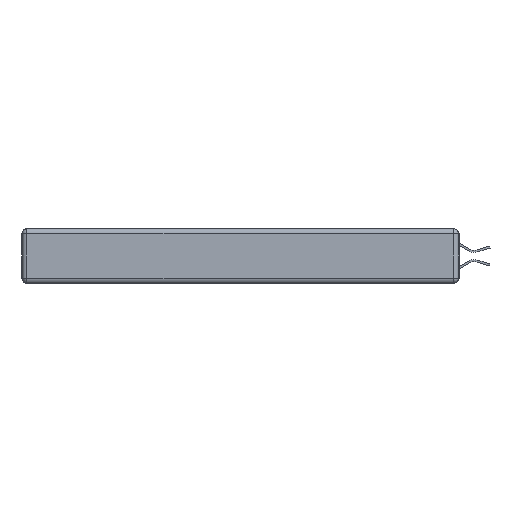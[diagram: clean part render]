
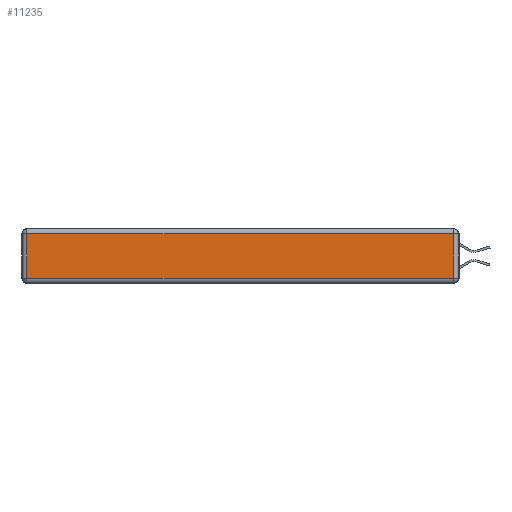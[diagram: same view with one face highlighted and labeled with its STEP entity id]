
A CAD part, left-side view. The second image highlights one B-rep face of the part: STEP entity #11235.
In plain terms, the highlighted planar face has unit normal (-1, 0, 0).
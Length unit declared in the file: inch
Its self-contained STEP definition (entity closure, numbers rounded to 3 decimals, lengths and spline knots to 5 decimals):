
#348 = VERTEX_POINT ( 'NONE', #9298 ) ;
#1305 = LINE ( 'NONE', #13973, #2367 ) ;
#1546 = ORIENTED_EDGE ( 'NONE', *, *, #17065, .T. ) ;
#2367 = VECTOR ( 'NONE', #12504, 39.37008 ) ;
#2488 = PLANE ( 'NONE',  #15989 ) ;
#2818 = VERTEX_POINT ( 'NONE', #19683 ) ;
#3318 = LINE ( 'NONE', #5672, #21257 ) ;
#3895 = FACE_OUTER_BOUND ( 'NONE', #20191, .T. ) ;
#5672 = CARTESIAN_POINT ( 'NONE',  ( 0., 2.75, -0.03 ) ) ;
#5924 = ORIENTED_EDGE ( 'NONE', *, *, #8957, .T. ) ;
#7052 = CARTESIAN_POINT ( 'NONE',  ( 0., 0., -0.313 ) ) ;
#7129 = DIRECTION ( 'NONE',  ( 0., -1., 0. ) ) ;
#7643 = ORIENTED_EDGE ( 'NONE', *, *, #12634, .T. ) ;
#8957 = EDGE_CURVE ( 'NONE', #348, #16930, #9731, .T. ) ;
#9298 = CARTESIAN_POINT ( 'NONE',  ( 0., 2.72, -0.313 ) ) ;
#9731 = LINE ( 'NONE', #7052, #20865 ) ;
#10136 = LINE ( 'NONE', #15287, #15699 ) ;
#10509 = EDGE_CURVE ( 'NONE', #16930, #14102, #1305, .T. ) ;
#11235 = ADVANCED_FACE ( 'NONE', ( #3895 ), #2488, .T. ) ;
#11899 = ORIENTED_EDGE ( 'NONE', *, *, #10509, .T. ) ;
#12504 = DIRECTION ( 'NONE',  ( 0., 0., 1. ) ) ;
#12634 = EDGE_CURVE ( 'NONE', #14102, #2818, #3318, .T. ) ;
#13973 = CARTESIAN_POINT ( 'NONE',  ( 0., 0.03, -0.343 ) ) ;
#14102 = VERTEX_POINT ( 'NONE', #19159 ) ;
#15287 = CARTESIAN_POINT ( 'NONE',  ( 0., 2.72, -0.343 ) ) ;
#15423 = DIRECTION ( 'NONE',  ( 0., 0., -1. ) ) ;
#15698 = DIRECTION ( 'NONE',  ( 0., 1., 0. ) ) ;
#15699 = VECTOR ( 'NONE', #15423, 39.37008 ) ;
#15709 = DIRECTION ( 'NONE',  ( -1., 0., 0. ) ) ;
#15989 = AXIS2_PLACEMENT_3D ( 'NONE', #19424, #15709, #21256 ) ;
#16930 = VERTEX_POINT ( 'NONE', #20160 ) ;
#17065 = EDGE_CURVE ( 'NONE', #2818, #348, #10136, .T. ) ;
#19159 = CARTESIAN_POINT ( 'NONE',  ( 0., 0.03, -0.03 ) ) ;
#19424 = CARTESIAN_POINT ( 'NONE',  ( 0., 0., -0.343 ) ) ;
#19683 = CARTESIAN_POINT ( 'NONE',  ( 0., 2.72, -0.03 ) ) ;
#20160 = CARTESIAN_POINT ( 'NONE',  ( 0., 0.03, -0.313 ) ) ;
#20191 = EDGE_LOOP ( 'NONE', ( #5924, #11899, #7643, #1546 ) ) ;
#20865 = VECTOR ( 'NONE', #7129, 39.37008 ) ;
#21256 = DIRECTION ( 'NONE',  ( 0., 0., 1. ) ) ;
#21257 = VECTOR ( 'NONE', #15698, 39.37008 ) ;
